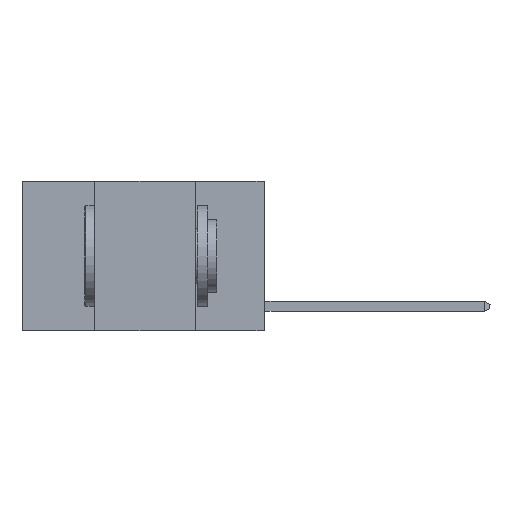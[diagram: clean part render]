
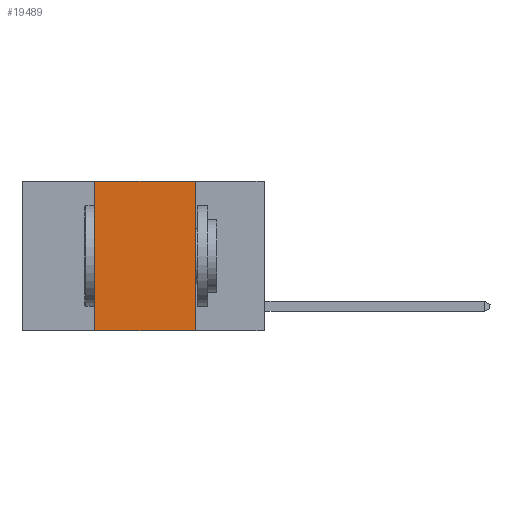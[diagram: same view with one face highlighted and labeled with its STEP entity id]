
A CAD part, left-side view. The second image highlights one B-rep face of the part: STEP entity #19489.
In plain terms, the highlighted planar face has unit normal (-1, 0, 0).
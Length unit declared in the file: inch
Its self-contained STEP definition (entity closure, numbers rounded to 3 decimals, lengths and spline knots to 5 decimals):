
#197 = ORIENTED_EDGE ( 'NONE', *, *, #22016, .T. ) ;
#629 = VERTEX_POINT ( 'NONE', #6538 ) ;
#2266 = LINE ( 'NONE', #4238, #8484 ) ;
#3771 = AXIS2_PLACEMENT_3D ( 'NONE', #15944, #7326, #6910 ) ;
#4238 = CARTESIAN_POINT ( 'NONE',  ( 0., 0.6, -0.37 ) ) ;
#4375 = DIRECTION ( 'NONE',  ( 0., -1., 0. ) ) ;
#5881 = CARTESIAN_POINT ( 'NONE',  ( 0., 0.6, 0. ) ) ;
#5968 = VECTOR ( 'NONE', #14374, 39.37008 ) ;
#6538 = CARTESIAN_POINT ( 'NONE',  ( 0., 0.42, 0. ) ) ;
#6910 = DIRECTION ( 'NONE',  ( 0., 0., -1. ) ) ;
#7046 = LINE ( 'NONE', #5881, #5968 ) ;
#7326 = DIRECTION ( 'NONE',  ( 1., 0., 0. ) ) ;
#7343 = ORIENTED_EDGE ( 'NONE', *, *, #26349, .F. ) ;
#8006 = LINE ( 'NONE', #20841, #9595 ) ;
#8484 = VECTOR ( 'NONE', #4375, 39.37008 ) ;
#9332 = CARTESIAN_POINT ( 'NONE',  ( 0., 0.17, -0.37 ) ) ;
#9595 = VECTOR ( 'NONE', #27293, 39.37008 ) ;
#9937 = CARTESIAN_POINT ( 'NONE',  ( 0., 0.42, -0.37 ) ) ;
#11241 = VECTOR ( 'NONE', #15680, 39.37008 ) ;
#11722 = LINE ( 'NONE', #20168, #11241 ) ;
#13356 = VERTEX_POINT ( 'NONE', #13844 ) ;
#13399 = EDGE_CURVE ( 'NONE', #21090, #629, #11722, .T. ) ;
#13844 = CARTESIAN_POINT ( 'NONE',  ( 0., 0.17, 0. ) ) ;
#14020 = ORIENTED_EDGE ( 'NONE', *, *, #13399, .F. ) ;
#14374 = DIRECTION ( 'NONE',  ( 0., -1., 0. ) ) ;
#15680 = DIRECTION ( 'NONE',  ( 0., 0., 1. ) ) ;
#15944 = CARTESIAN_POINT ( 'NONE',  ( 0., 0.6, 0. ) ) ;
#18758 = ORIENTED_EDGE ( 'NONE', *, *, #26300, .F. ) ;
#19489 = ADVANCED_FACE ( 'NONE', ( #25630 ), #21428, .F. ) ;
#20168 = CARTESIAN_POINT ( 'NONE',  ( 0., 0.42, 0. ) ) ;
#20841 = CARTESIAN_POINT ( 'NONE',  ( 0., 0.17, 0. ) ) ;
#21090 = VERTEX_POINT ( 'NONE', #9937 ) ;
#21428 = PLANE ( 'NONE',  #3771 ) ;
#22016 = EDGE_CURVE ( 'NONE', #21090, #27679, #2266, .T. ) ;
#25630 = FACE_OUTER_BOUND ( 'NONE', #26927, .T. ) ;
#26300 = EDGE_CURVE ( 'NONE', #629, #13356, #7046, .T. ) ;
#26349 = EDGE_CURVE ( 'NONE', #13356, #27679, #8006, .T. ) ;
#26927 = EDGE_LOOP ( 'NONE', ( #7343, #18758, #14020, #197 ) ) ;
#27293 = DIRECTION ( 'NONE',  ( 0., 0., -1. ) ) ;
#27679 = VERTEX_POINT ( 'NONE', #9332 ) ;
